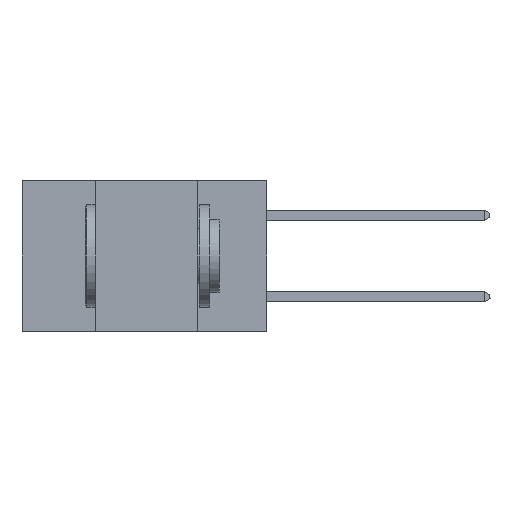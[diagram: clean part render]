
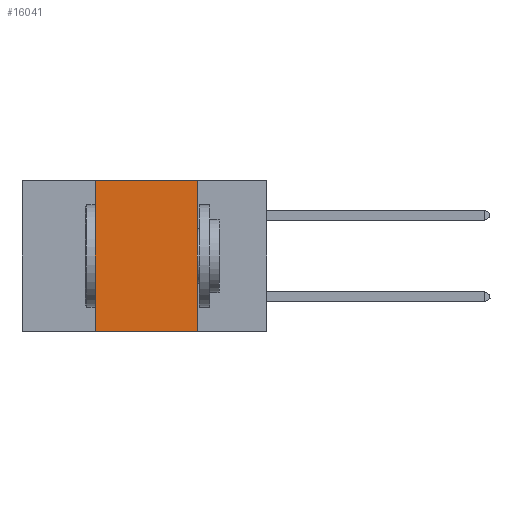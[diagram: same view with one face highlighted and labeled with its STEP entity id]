
A CAD part, left-side view. The second image highlights one B-rep face of the part: STEP entity #16041.
In plain terms, the highlighted planar face has unit normal (-1, 0, 0).
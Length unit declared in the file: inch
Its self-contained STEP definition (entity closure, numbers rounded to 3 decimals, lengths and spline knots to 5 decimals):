
#714 = DIRECTION ( 'NONE',  ( 1., 0., 0. ) ) ;
#1376 = LINE ( 'NONE', #14102, #16916 ) ;
#1420 = EDGE_CURVE ( 'NONE', #17037, #16735, #6688, .T. ) ;
#2061 = DIRECTION ( 'NONE',  ( 0., 0., -1. ) ) ;
#2485 = CARTESIAN_POINT ( 'NONE',  ( 0., 0.42, 0. ) ) ;
#2639 = LINE ( 'NONE', #2485, #10683 ) ;
#2909 = ORIENTED_EDGE ( 'NONE', *, *, #14180, .F. ) ;
#3286 = VERTEX_POINT ( 'NONE', #11769 ) ;
#3834 = DIRECTION ( 'NONE',  ( 0., -1., 0. ) ) ;
#4148 = CARTESIAN_POINT ( 'NONE',  ( 0., 0.6, -0.37 ) ) ;
#6486 = CARTESIAN_POINT ( 'NONE',  ( 0., 0.42, 0. ) ) ;
#6688 = LINE ( 'NONE', #4148, #10175 ) ;
#8635 = FACE_OUTER_BOUND ( 'NONE', #19272, .T. ) ;
#8845 = VERTEX_POINT ( 'NONE', #6486 ) ;
#9684 = CARTESIAN_POINT ( 'NONE',  ( 0., 0.17, 0. ) ) ;
#10175 = VECTOR ( 'NONE', #3834, 39.37008 ) ;
#10683 = VECTOR ( 'NONE', #11541, 39.37008 ) ;
#11387 = DIRECTION ( 'NONE',  ( 0., 0., -1. ) ) ;
#11415 = ORIENTED_EDGE ( 'NONE', *, *, #13676, .F. ) ;
#11541 = DIRECTION ( 'NONE',  ( 0., 0., 1. ) ) ;
#11769 = CARTESIAN_POINT ( 'NONE',  ( 0., 0.17, 0. ) ) ;
#12469 = AXIS2_PLACEMENT_3D ( 'NONE', #12823, #714, #11387 ) ;
#12823 = CARTESIAN_POINT ( 'NONE',  ( 0., 0.6, 0. ) ) ;
#13676 = EDGE_CURVE ( 'NONE', #17037, #8845, #2639, .T. ) ;
#13863 = LINE ( 'NONE', #9684, #17321 ) ;
#14102 = CARTESIAN_POINT ( 'NONE',  ( 0., 0.6, 0. ) ) ;
#14163 = DIRECTION ( 'NONE',  ( 0., -1., 0. ) ) ;
#14180 = EDGE_CURVE ( 'NONE', #8845, #3286, #1376, .T. ) ;
#14418 = ORIENTED_EDGE ( 'NONE', *, *, #19192, .F. ) ;
#15331 = ORIENTED_EDGE ( 'NONE', *, *, #1420, .T. ) ;
#15767 = PLANE ( 'NONE',  #12469 ) ;
#16041 = ADVANCED_FACE ( 'NONE', ( #8635 ), #15767, .F. ) ;
#16735 = VERTEX_POINT ( 'NONE', #18528 ) ;
#16916 = VECTOR ( 'NONE', #14163, 39.37008 ) ;
#17037 = VERTEX_POINT ( 'NONE', #18142 ) ;
#17321 = VECTOR ( 'NONE', #2061, 39.37008 ) ;
#18142 = CARTESIAN_POINT ( 'NONE',  ( 0., 0.42, -0.37 ) ) ;
#18528 = CARTESIAN_POINT ( 'NONE',  ( 0., 0.17, -0.37 ) ) ;
#19192 = EDGE_CURVE ( 'NONE', #3286, #16735, #13863, .T. ) ;
#19272 = EDGE_LOOP ( 'NONE', ( #14418, #2909, #11415, #15331 ) ) ;
